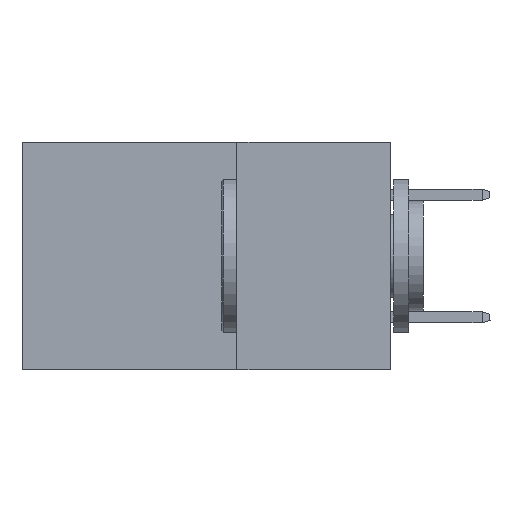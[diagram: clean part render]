
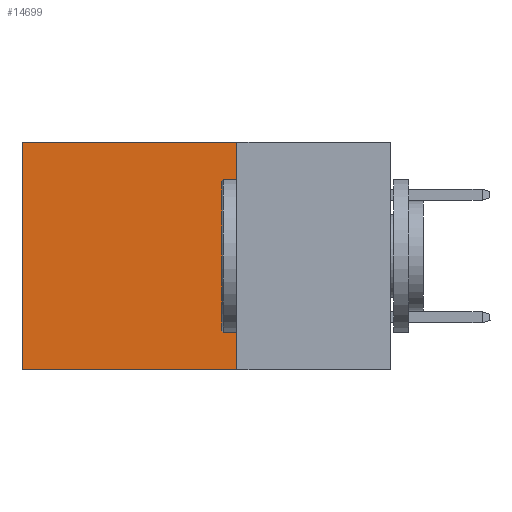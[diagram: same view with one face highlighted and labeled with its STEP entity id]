
A CAD part, left-side view. The second image highlights one B-rep face of the part: STEP entity #14699.
In plain terms, the highlighted planar face has unit normal (-1, 0, 0).
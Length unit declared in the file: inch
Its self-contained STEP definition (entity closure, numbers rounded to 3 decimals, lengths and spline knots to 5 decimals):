
#735 = CARTESIAN_POINT ( 'NONE',  ( 0.2875, 0.25, -0.37 ) ) ;
#898 = VERTEX_POINT ( 'NONE', #9456 ) ;
#1198 = CARTESIAN_POINT ( 'NONE',  ( 0.2875, 0.6, 0. ) ) ;
#1562 = ORIENTED_EDGE ( 'NONE', *, *, #2333, .F. ) ;
#2014 = LINE ( 'NONE', #2922, #15498 ) ;
#2333 = EDGE_CURVE ( 'NONE', #898, #13501, #10148, .T. ) ;
#2868 = VECTOR ( 'NONE', #11759, 39.37008 ) ;
#2922 = CARTESIAN_POINT ( 'NONE',  ( 0.2875, 0.6, 0. ) ) ;
#2953 = VECTOR ( 'NONE', #11287, 39.37008 ) ;
#3138 = DIRECTION ( 'NONE',  ( 1., 0., 0. ) ) ;
#4294 = DIRECTION ( 'NONE',  ( 0., 0., -1. ) ) ;
#4501 = DIRECTION ( 'NONE',  ( 0., 0., -1. ) ) ;
#4900 = EDGE_CURVE ( 'NONE', #9531, #13501, #2014, .T. ) ;
#5261 = EDGE_CURVE ( 'NONE', #6014, #9531, #13648, .T. ) ;
#5385 = LINE ( 'NONE', #13937, #15224 ) ;
#5982 = CARTESIAN_POINT ( 'NONE',  ( 0.2875, 0.6, -0.37 ) ) ;
#6014 = VERTEX_POINT ( 'NONE', #15876 ) ;
#9456 = CARTESIAN_POINT ( 'NONE',  ( 0.2875, 0.25, -0.37 ) ) ;
#9531 = VERTEX_POINT ( 'NONE', #1198 ) ;
#9861 = PLANE ( 'NONE',  #15524 ) ;
#9888 = ORIENTED_EDGE ( 'NONE', *, *, #4900, .T. ) ;
#10148 = LINE ( 'NONE', #735, #2953 ) ;
#10437 = CARTESIAN_POINT ( 'NONE',  ( 0.2875, 0.25, 0. ) ) ;
#10823 = EDGE_LOOP ( 'NONE', ( #9888, #1562, #13603, #13742 ) ) ;
#11287 = DIRECTION ( 'NONE',  ( 0., 1., 0. ) ) ;
#11759 = DIRECTION ( 'NONE',  ( 0., 1., 0. ) ) ;
#12092 = FACE_OUTER_BOUND ( 'NONE', #10823, .T. ) ;
#12558 = DIRECTION ( 'NONE',  ( 0., 0., -1. ) ) ;
#13501 = VERTEX_POINT ( 'NONE', #5982 ) ;
#13603 = ORIENTED_EDGE ( 'NONE', *, *, #14708, .F. ) ;
#13648 = LINE ( 'NONE', #10437, #2868 ) ;
#13742 = ORIENTED_EDGE ( 'NONE', *, *, #5261, .T. ) ;
#13937 = CARTESIAN_POINT ( 'NONE',  ( 0.2875, 0.25, 0. ) ) ;
#14699 = ADVANCED_FACE ( 'NONE', ( #12092 ), #9861, .F. ) ;
#14708 = EDGE_CURVE ( 'NONE', #6014, #898, #5385, .T. ) ;
#15120 = CARTESIAN_POINT ( 'NONE',  ( 0.2875, 0.25, 0. ) ) ;
#15224 = VECTOR ( 'NONE', #4501, 39.37008 ) ;
#15498 = VECTOR ( 'NONE', #4294, 39.37008 ) ;
#15524 = AXIS2_PLACEMENT_3D ( 'NONE', #15120, #3138, #12558 ) ;
#15876 = CARTESIAN_POINT ( 'NONE',  ( 0.2875, 0.25, 0. ) ) ;
